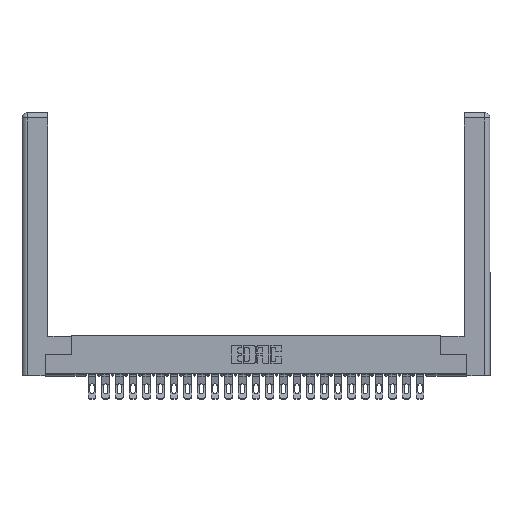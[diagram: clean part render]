
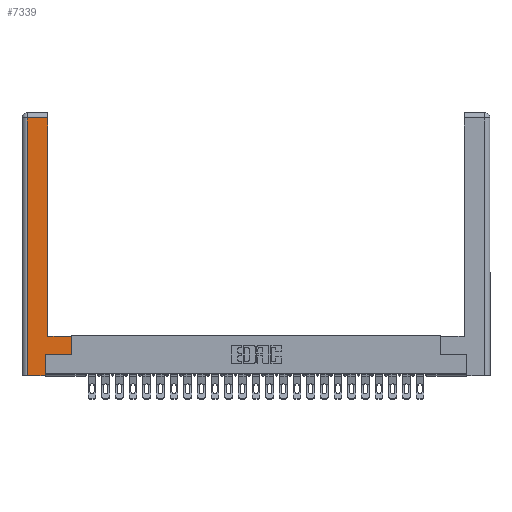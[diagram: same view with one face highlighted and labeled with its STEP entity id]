
A CAD part, top view. The second image highlights one B-rep face of the part: STEP entity #7339.
In plain terms, the highlighted planar face has unit normal (0, 0, 1).
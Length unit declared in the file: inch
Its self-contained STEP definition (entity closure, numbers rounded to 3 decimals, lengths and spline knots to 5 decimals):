
#24 = EDGE_CURVE ( 'NONE', #11255, #30991, #12771, .T. ) ;
#170 = EDGE_CURVE ( 'NONE', #14641, #11255, #22192, .T. ) ;
#804 = CARTESIAN_POINT ( 'NONE',  ( 0.565, 0.45, 0. ) ) ;
#1816 = CARTESIAN_POINT ( 'NONE',  ( 0.265, 0., 0. ) ) ;
#2490 = CARTESIAN_POINT ( 'NONE',  ( 0.295, 0.45, 0. ) ) ;
#2504 = CARTESIAN_POINT ( 'NONE',  ( 0.0615, 2.94, 0. ) ) ;
#2701 = EDGE_CURVE ( 'NONE', #6016, #4064, #5220, .T. ) ;
#3205 = ORIENTED_EDGE ( 'NONE', *, *, #2701, .T. ) ;
#4064 = VERTEX_POINT ( 'NONE', #8625 ) ;
#4621 = VECTOR ( 'NONE', #16509, 39.37008 ) ;
#5220 = LINE ( 'NONE', #18737, #11076 ) ;
#5654 = LINE ( 'NONE', #2490, #18189 ) ;
#5834 = ORIENTED_EDGE ( 'NONE', *, *, #6665, .T. ) ;
#6016 = VERTEX_POINT ( 'NONE', #9519 ) ;
#6665 = EDGE_CURVE ( 'NONE', #4064, #22529, #29815, .T. ) ;
#7284 = CARTESIAN_POINT ( 'NONE',  ( 0.0615, 0., 0. ) ) ;
#7339 = ADVANCED_FACE ( 'NONE', ( #27437 ), #12373, .F. ) ;
#7407 = CARTESIAN_POINT ( 'NONE',  ( 0.265, 0.245, 0. ) ) ;
#7805 = ORIENTED_EDGE ( 'NONE', *, *, #21573, .T. ) ;
#8625 = CARTESIAN_POINT ( 'NONE',  ( 0.295, 2.94, 0. ) ) ;
#8884 = VECTOR ( 'NONE', #17527, 39.37008 ) ;
#9386 = ORIENTED_EDGE ( 'NONE', *, *, #170, .T. ) ;
#9519 = CARTESIAN_POINT ( 'NONE',  ( 0.295, 0.45, 0. ) ) ;
#10686 = EDGE_CURVE ( 'NONE', #22529, #23041, #22896, .T. ) ;
#11076 = VECTOR ( 'NONE', #16507, 39.37008 ) ;
#11255 = VERTEX_POINT ( 'NONE', #26861 ) ;
#12373 = PLANE ( 'NONE',  #17613 ) ;
#12609 = CARTESIAN_POINT ( 'NONE',  ( 0.565, 0.245, 0. ) ) ;
#12771 = LINE ( 'NONE', #804, #25296 ) ;
#12779 = ORIENTED_EDGE ( 'NONE', *, *, #26670, .T. ) ;
#13887 = CARTESIAN_POINT ( 'NONE',  ( 0.265, 0., 0. ) ) ;
#14632 = DIRECTION ( 'NONE',  ( 0., 0., -1. ) ) ;
#14641 = VERTEX_POINT ( 'NONE', #7407 ) ;
#15136 = EDGE_CURVE ( 'NONE', #23041, #19690, #26198, .T. ) ;
#16172 = DIRECTION ( 'NONE',  ( -1., 0., 0. ) ) ;
#16507 = DIRECTION ( 'NONE',  ( 0., 1., 0. ) ) ;
#16509 = DIRECTION ( 'NONE',  ( 0., 1., 0. ) ) ;
#17527 = DIRECTION ( 'NONE',  ( 1., 0., 0. ) ) ;
#17613 = AXIS2_PLACEMENT_3D ( 'NONE', #24744, #14632, #22444 ) ;
#17873 = CARTESIAN_POINT ( 'NONE',  ( 0.565, 0.45, 0. ) ) ;
#18091 = VECTOR ( 'NONE', #16172, 39.37008 ) ;
#18176 = CARTESIAN_POINT ( 'NONE',  ( 0.0615, 0., 0. ) ) ;
#18189 = VECTOR ( 'NONE', #22619, 39.37008 ) ;
#18737 = CARTESIAN_POINT ( 'NONE',  ( 0.295, 3., 0. ) ) ;
#19338 = DIRECTION ( 'NONE',  ( 1., 0., 0. ) ) ;
#19690 = VERTEX_POINT ( 'NONE', #13887 ) ;
#20807 = DIRECTION ( 'NONE',  ( 0., -1., 0. ) ) ;
#21573 = EDGE_CURVE ( 'NONE', #19690, #14641, #31250, .T. ) ;
#22058 = EDGE_LOOP ( 'NONE', ( #3205, #5834, #29066, #29261, #7805, #9386, #28996, #12779 ) ) ;
#22192 = LINE ( 'NONE', #12609, #8884 ) ;
#22444 = DIRECTION ( 'NONE',  ( -1., 0., 0. ) ) ;
#22529 = VERTEX_POINT ( 'NONE', #2504 ) ;
#22619 = DIRECTION ( 'NONE',  ( -1., 0., 0. ) ) ;
#22896 = LINE ( 'NONE', #18176, #26027 ) ;
#23041 = VERTEX_POINT ( 'NONE', #7284 ) ;
#24744 = CARTESIAN_POINT ( 'NONE',  ( 0., 0., 0. ) ) ;
#25296 = VECTOR ( 'NONE', #27269, 39.37008 ) ;
#26027 = VECTOR ( 'NONE', #20807, 39.37008 ) ;
#26198 = LINE ( 'NONE', #1816, #30493 ) ;
#26670 = EDGE_CURVE ( 'NONE', #30991, #6016, #5654, .T. ) ;
#26861 = CARTESIAN_POINT ( 'NONE',  ( 0.565, 0.245, 0. ) ) ;
#27269 = DIRECTION ( 'NONE',  ( 0., 1., 0. ) ) ;
#27437 = FACE_OUTER_BOUND ( 'NONE', #22058, .T. ) ;
#28653 = CARTESIAN_POINT ( 'NONE',  ( 0.265, 0.245, 0. ) ) ;
#28996 = ORIENTED_EDGE ( 'NONE', *, *, #24, .T. ) ;
#29066 = ORIENTED_EDGE ( 'NONE', *, *, #10686, .T. ) ;
#29261 = ORIENTED_EDGE ( 'NONE', *, *, #15136, .T. ) ;
#29815 = LINE ( 'NONE', #31063, #18091 ) ;
#30493 = VECTOR ( 'NONE', #19338, 39.37008 ) ;
#30991 = VERTEX_POINT ( 'NONE', #17873 ) ;
#31063 = CARTESIAN_POINT ( 'NONE',  ( 0.0615, 2.94, 0. ) ) ;
#31250 = LINE ( 'NONE', #28653, #4621 ) ;
